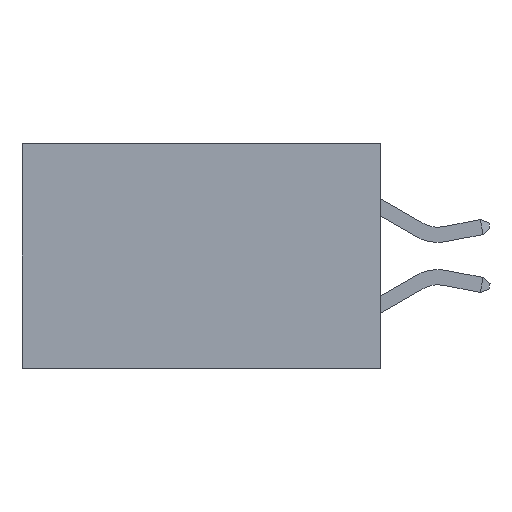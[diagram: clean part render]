
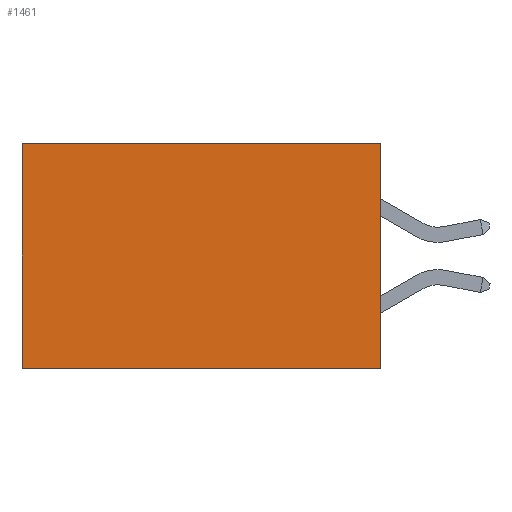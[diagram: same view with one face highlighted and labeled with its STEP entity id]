
A CAD part, left-side view. The second image highlights one B-rep face of the part: STEP entity #1461.
In plain terms, the highlighted planar face has unit normal (-1, 0, 0).
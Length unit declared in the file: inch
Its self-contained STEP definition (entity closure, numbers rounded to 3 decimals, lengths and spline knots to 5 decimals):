
#156 = CARTESIAN_POINT ( 'NONE',  ( 0.277, 0., -0.37 ) ) ;
#281 = AXIS2_PLACEMENT_3D ( 'NONE', #156, #2484, #7491 ) ;
#282 = VERTEX_POINT ( 'NONE', #10952 ) ;
#438 = LINE ( 'NONE', #4002, #5764 ) ;
#539 = FACE_OUTER_BOUND ( 'NONE', #11527, .T. ) ;
#1028 = DIRECTION ( 'NONE',  ( 0., 0., -1. ) ) ;
#1330 = VECTOR ( 'NONE', #6927, 39.37008 ) ;
#1366 = VERTEX_POINT ( 'NONE', #4320 ) ;
#1461 = ADVANCED_FACE ( 'NONE', ( #539 ), #12981, .F. ) ;
#2484 = DIRECTION ( 'NONE',  ( 1., 0., 0. ) ) ;
#2755 = ORIENTED_EDGE ( 'NONE', *, *, #10597, .F. ) ;
#3939 = DIRECTION ( 'NONE',  ( 0., 1., 0. ) ) ;
#4002 = CARTESIAN_POINT ( 'NONE',  ( 0.277, 0., -0.37 ) ) ;
#4226 = CARTESIAN_POINT ( 'NONE',  ( 0.277, 0., -0.37 ) ) ;
#4320 = CARTESIAN_POINT ( 'NONE',  ( 0.277, 0.59, 0. ) ) ;
#4493 = VERTEX_POINT ( 'NONE', #10430 ) ;
#4797 = CARTESIAN_POINT ( 'NONE',  ( 0.277, 0.59, -0.37 ) ) ;
#5213 = ORIENTED_EDGE ( 'NONE', *, *, #9464, .T. ) ;
#5287 = EDGE_CURVE ( 'NONE', #282, #9396, #438, .T. ) ;
#5522 = ORIENTED_EDGE ( 'NONE', *, *, #7523, .T. ) ;
#5764 = VECTOR ( 'NONE', #3939, 39.37008 ) ;
#6164 = LINE ( 'NONE', #4226, #11669 ) ;
#6927 = DIRECTION ( 'NONE',  ( 0., 1., 0. ) ) ;
#6973 = CARTESIAN_POINT ( 'NONE',  ( 0.277, 0., 0. ) ) ;
#7491 = DIRECTION ( 'NONE',  ( 0., 0., -1. ) ) ;
#7523 = EDGE_CURVE ( 'NONE', #4493, #1366, #12083, .T. ) ;
#7992 = CARTESIAN_POINT ( 'NONE',  ( 0.277, 0.59, -0.37 ) ) ;
#7993 = ORIENTED_EDGE ( 'NONE', *, *, #5287, .F. ) ;
#9064 = DIRECTION ( 'NONE',  ( 0., 0., -1. ) ) ;
#9396 = VERTEX_POINT ( 'NONE', #4797 ) ;
#9464 = EDGE_CURVE ( 'NONE', #1366, #9396, #13108, .T. ) ;
#10430 = CARTESIAN_POINT ( 'NONE',  ( 0.277, 0., 0. ) ) ;
#10451 = VECTOR ( 'NONE', #9064, 39.37008 ) ;
#10597 = EDGE_CURVE ( 'NONE', #4493, #282, #6164, .T. ) ;
#10952 = CARTESIAN_POINT ( 'NONE',  ( 0.277, 0., -0.37 ) ) ;
#11527 = EDGE_LOOP ( 'NONE', ( #5213, #7993, #2755, #5522 ) ) ;
#11669 = VECTOR ( 'NONE', #1028, 39.37008 ) ;
#12083 = LINE ( 'NONE', #6973, #1330 ) ;
#12981 = PLANE ( 'NONE',  #281 ) ;
#13108 = LINE ( 'NONE', #7992, #10451 ) ;
